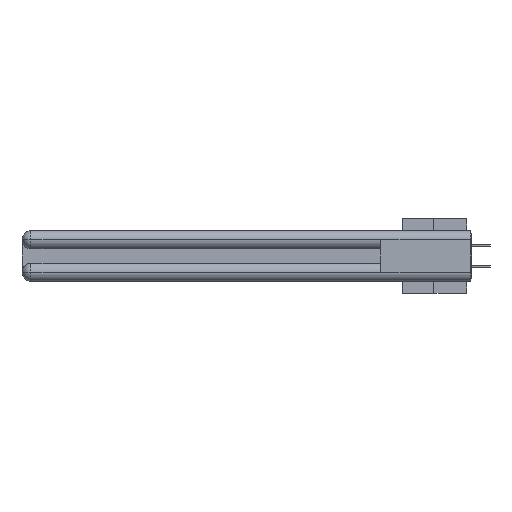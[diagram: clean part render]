
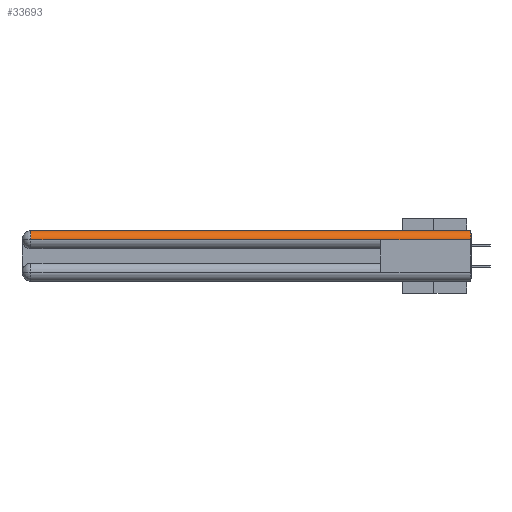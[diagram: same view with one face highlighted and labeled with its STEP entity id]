
A CAD part, left-side view. The second image highlights one B-rep face of the part: STEP entity #33693.
In plain terms, the highlighted cylindrical face has radius 1.562 mm (diameter 3.124 mm), a partial arc.
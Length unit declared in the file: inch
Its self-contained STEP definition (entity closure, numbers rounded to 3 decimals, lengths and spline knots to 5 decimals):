
#267 = DIRECTION ( 'NONE',  ( 0., -1., 0. ) ) ;
#346 = AXIS2_PLACEMENT_3D ( 'NONE', #36949, #13585, #33853 ) ;
#2407 = ORIENTED_EDGE ( 'NONE', *, *, #30601, .F. ) ;
#3491 = VECTOR ( 'NONE', #35491, 39.37008 ) ;
#3848 = CYLINDRICAL_SURFACE ( 'NONE', #29510, 0.0615 ) ;
#4059 = ORIENTED_EDGE ( 'NONE', *, *, #25219, .F. ) ;
#4231 = VECTOR ( 'NONE', #35279, 39.37008 ) ;
#4822 = FACE_OUTER_BOUND ( 'NONE', #28222, .T. ) ;
#5620 = CIRCLE ( 'NONE', #13712, 0.0615 ) ;
#6454 = CARTESIAN_POINT ( 'NONE',  ( 0., 2.94, -0.0615 ) ) ;
#6669 = EDGE_CURVE ( 'NONE', #13539, #7435, #5620, .T. ) ;
#6953 = CARTESIAN_POINT ( 'NONE',  ( 0.0615, 0., -0.0615 ) ) ;
#7410 = VECTOR ( 'NONE', #267, 39.37008 ) ;
#7435 = VERTEX_POINT ( 'NONE', #11171 ) ;
#8232 = ORIENTED_EDGE ( 'NONE', *, *, #35392, .T. ) ;
#8359 = LINE ( 'NONE', #22483, #4231 ) ;
#8527 = DIRECTION ( 'NONE',  ( 1., 0., 0. ) ) ;
#8605 = LINE ( 'NONE', #8797, #3491 ) ;
#8797 = CARTESIAN_POINT ( 'NONE',  ( 0., 3., -0.0615 ) ) ;
#9202 = ORIENTED_EDGE ( 'NONE', *, *, #6669, .F. ) ;
#11171 = CARTESIAN_POINT ( 'NONE',  ( 0., 0., -0.0615 ) ) ;
#13539 = VERTEX_POINT ( 'NONE', #21262 ) ;
#13585 = DIRECTION ( 'NONE',  ( 0., -1., 0. ) ) ;
#13712 = AXIS2_PLACEMENT_3D ( 'NONE', #21287, #18346, #8527 ) ;
#13884 = EDGE_CURVE ( 'NONE', #20861, #36059, #15146, .T. ) ;
#14774 = LINE ( 'NONE', #29761, #7410 ) ;
#15146 = CIRCLE ( 'NONE', #346, 0.0615 ) ;
#18346 = DIRECTION ( 'NONE',  ( 0., -1., 0. ) ) ;
#20861 = VERTEX_POINT ( 'NONE', #35842 ) ;
#21262 = CARTESIAN_POINT ( 'NONE',  ( 0.0615, 0., 0. ) ) ;
#21287 = CARTESIAN_POINT ( 'NONE',  ( 0.0615, 0., -0.0615 ) ) ;
#22264 = DIRECTION ( 'NONE',  ( 0., 0., 1. ) ) ;
#22483 = CARTESIAN_POINT ( 'NONE',  ( 0., 3., -0.0615 ) ) ;
#24043 = ORIENTED_EDGE ( 'NONE', *, *, #13884, .T. ) ;
#25219 = EDGE_CURVE ( 'NONE', #7435, #35414, #8605, .T. ) ;
#26419 = CARTESIAN_POINT ( 'NONE',  ( 0., 0.6, -0.0615 ) ) ;
#28222 = EDGE_LOOP ( 'NONE', ( #2407, #24043, #8232, #4059, #9202 ) ) ;
#29510 = AXIS2_PLACEMENT_3D ( 'NONE', #6953, #36735, #22264 ) ;
#29761 = CARTESIAN_POINT ( 'NONE',  ( 0.0615, 0., 0. ) ) ;
#30601 = EDGE_CURVE ( 'NONE', #20861, #13539, #14774, .T. ) ;
#33693 = ADVANCED_FACE ( 'NONE', ( #4822 ), #3848, .T. ) ;
#33853 = DIRECTION ( 'NONE',  ( 0., 0., 1. ) ) ;
#35279 = DIRECTION ( 'NONE',  ( 0., -1., 0. ) ) ;
#35392 = EDGE_CURVE ( 'NONE', #36059, #35414, #8359, .T. ) ;
#35414 = VERTEX_POINT ( 'NONE', #26419 ) ;
#35491 = DIRECTION ( 'NONE',  ( 0., 1., 0. ) ) ;
#35842 = CARTESIAN_POINT ( 'NONE',  ( 0.0615, 2.94, 0. ) ) ;
#36059 = VERTEX_POINT ( 'NONE', #6454 ) ;
#36735 = DIRECTION ( 'NONE',  ( 0., 1., 0. ) ) ;
#36949 = CARTESIAN_POINT ( 'NONE',  ( 0.0615, 2.94, -0.0615 ) ) ;
